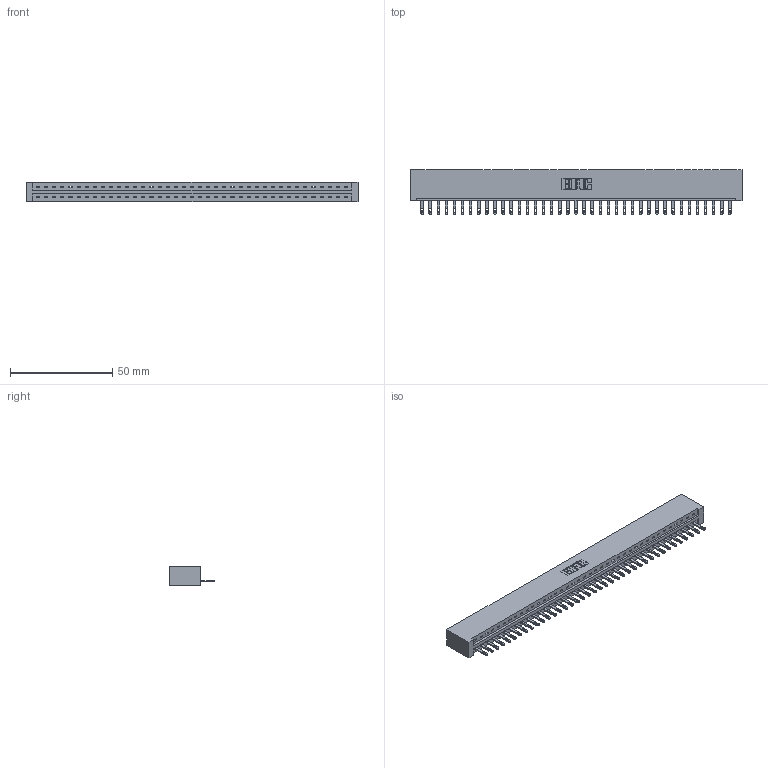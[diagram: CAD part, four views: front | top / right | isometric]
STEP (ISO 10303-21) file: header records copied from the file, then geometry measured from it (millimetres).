
FILE_DESCRIPTION (( 'STEP AP203' ), '1' );
FILE_NAME ('337-039-500-101.STEP', '2018-08-08T06:26:48', ( '' ), ( '' ), 'SwSTEP 2.0', 'SolidWorks 2016', '' );
FILE_SCHEMA (( 'CONFIG_CONTROL_DESIGN' ));
Length unit declared in the file: inch
Products named in the file (3): 337-039-500-101; 337 Part_No Mounting Lugs; 345-292-001_345-293-100
Assembly tree (40 placements, depth 2):
  337-039-500-101
    337 Part_No Mounting Lugs
    345-292-001_345-293-100  x39
Bounding box: 162.41 x 21.85 x 9.4 mm (x, y, z)
Volume: 17604.9 mm3; surface area: 18247.9 mm2
Topology: 40 solids, 40 shells, 2368 faces, 7307 edges, 4870 vertices
Faces by surface type: plane 1626, cylinder 742
Entity records: 29031 total; most frequent: CARTESIAN_POINT 5063, ORIENTED_EDGE 5038, DIRECTION 4261, EDGE_CURVE 2519, LINE 2395, VECTOR 2395, VERTEX_POINT 1678, AXIS2_PLACEMENT_3D 933
